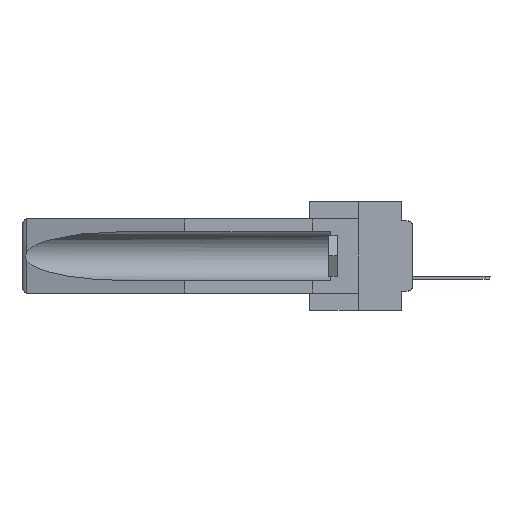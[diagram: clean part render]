
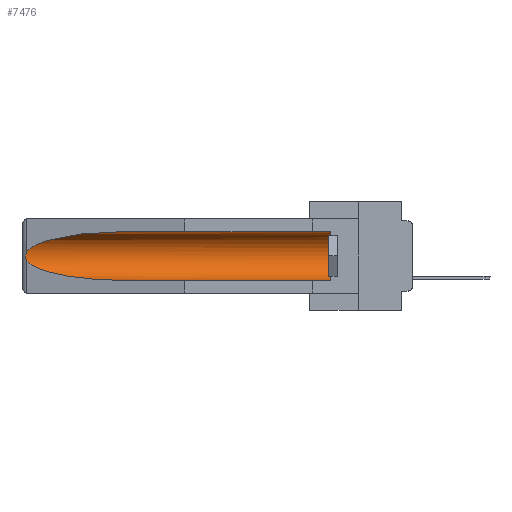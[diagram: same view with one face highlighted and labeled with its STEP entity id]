
A CAD part, left-side view. The second image highlights one B-rep face of the part: STEP entity #7476.
In plain terms, the highlighted cylindrical face has radius 2.857 mm (diameter 5.715 mm), a partial arc.
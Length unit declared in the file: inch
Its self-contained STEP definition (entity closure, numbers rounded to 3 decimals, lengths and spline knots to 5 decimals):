
#289 = VERTEX_POINT ( 'NONE', #1878 ) ;
#341 = DIRECTION ( 'NONE',  ( 0., 0., 1. ) ) ;
#725 = LINE ( 'NONE', #33284, #6023 ) ;
#1368 = ORIENTED_EDGE ( 'NONE', *, *, #16022, .T. ) ;
#1583 = EDGE_CURVE ( 'NONE', #289, #24981, #30473, .T. ) ;
#1784 = CARTESIAN_POINT ( 'NONE',  ( 0.155, 1.07973, -0.284 ) ) ;
#1878 = CARTESIAN_POINT ( 'NONE',  ( 0.155, 1.07973, -0.059 ) ) ;
#2144 = CARTESIAN_POINT ( 'NONE',  ( 0.2675, 1.53308, -0.16763 ) ) ;
#2725 = EDGE_LOOP ( 'NONE', ( #32180, #23673, #1368, #21050, #5216, #3379 ) ) ;
#2933 = EDGE_CURVE ( 'NONE', #29592, #12455, #725, .T. ) ;
#3379 = ORIENTED_EDGE ( 'NONE', *, *, #3585, .T. ) ;
#3585 = EDGE_CURVE ( 'NONE', #12005, #289, #24762, .T. ) ;
#5216 = ORIENTED_EDGE ( 'NONE', *, *, #14655, .T. ) ;
#6023 = VECTOR ( 'NONE', #20231, 39.37008 ) ;
#7077 = CARTESIAN_POINT ( 'NONE',  ( 0.155, 0.126, -0.059 ) ) ;
#7353 = CARTESIAN_POINT ( 'NONE',  ( 0.26655, 1.53094, -0.18657 ) ) ;
#7474 = CARTESIAN_POINT ( 'NONE',  ( 0.2673, 1.53269, -0.17917 ) ) ;
#7476 = ADVANCED_FACE ( 'NONE', ( #9332 ), #32379, .F. ) ;
#8204 = CARTESIAN_POINT ( 'NONE',  ( 0.155, -0.30754, -0.059 ) ) ;
#9332 = FACE_OUTER_BOUND ( 'NONE', #2725, .T. ) ;
#9966 = CARTESIAN_POINT ( 'NONE',  ( 0.26537, 1.52718, -0.14972 ) ) ;
#10027 = CARTESIAN_POINT ( 'NONE',  ( 0.26537, 1.52718, -0.14972 ) ) ;
#10951 = DIRECTION ( 'NONE',  ( 0., 1., 0. ) ) ;
#11073 = CARTESIAN_POINT ( 'NONE',  ( 0.21114, 1.30732, -0.059 ) ) ;
#11259 = CARTESIAN_POINT ( 'NONE',  ( 0.155, 1.07973, -0.284 ) ) ;
#12005 = VERTEX_POINT ( 'NONE', #7077 ) ;
#12455 = VERTEX_POINT ( 'NONE', #1784 ) ;
#12849 = AXIS2_PLACEMENT_3D ( 'NONE', #22186, #17029, #16928 ) ;
#13623 = CIRCLE ( 'NONE', #12849, 0.1125 ) ;
#13941 = CARTESIAN_POINT ( 'NONE',  ( 0.26537, 1.52718, -0.14972 ) ) ;
#14138 = CARTESIAN_POINT ( 'NONE',  ( 0.25451, 1.48313, -0.24835 ) ) ;
#14655 = EDGE_CURVE ( 'NONE', #29592, #12005, #13623, .T. ) ;
#14914 = VECTOR ( 'NONE', #10951, 39.37008 ) ;
#15169 = CARTESIAN_POINT ( 'NONE',  ( 0.26537, 1.52718, -0.19328 ) ) ;
#16022 = EDGE_CURVE ( 'NONE', #21710, #12455, #29589, .T. ) ;
#16928 = DIRECTION ( 'NONE',  ( 0., 0., 1. ) ) ;
#17029 = DIRECTION ( 'NONE',  ( 0., -1., 0. ) ) ;
#19294 = CARTESIAN_POINT ( 'NONE',  ( 0.21114, 1.30732, -0.284 ) ) ;
#19414 = CARTESIAN_POINT ( 'NONE',  ( 0.26537, 1.52718, -0.19328 ) ) ;
#20231 = DIRECTION ( 'NONE',  ( 0., 1., 0. ) ) ;
#21050 = ORIENTED_EDGE ( 'NONE', *, *, #2933, .F. ) ;
#21710 = VERTEX_POINT ( 'NONE', #25976 ) ;
#22186 = CARTESIAN_POINT ( 'NONE',  ( 0.155, 0.126, -0.1715 ) ) ;
#22338 = CARTESIAN_POINT ( 'NONE',  ( 0.155, 0.126, -0.284 ) ) ;
#22827 = B_SPLINE_CURVE_WITH_KNOTS ( 'NONE', 3,
 ( #10027, #25744, #23201, #28521, #2144, #28415, #7474, #7353, #33934, #15169 ),
 .UNSPECIFIED., .F., .F.,
 ( 4, 2, 2, 2, 4 ),
 ( 0., 0.00029, 0.00058, 0.00087, 0.00117 ),
 .UNSPECIFIED. ) ;
#23201 = CARTESIAN_POINT ( 'NONE',  ( 0.26654, 1.53092, -0.15636 ) ) ;
#23425 = AXIS2_PLACEMENT_3D ( 'NONE', #26590, #29273, #341 ) ;
#23673 = ORIENTED_EDGE ( 'NONE', *, *, #28598, .T. ) ;
#24762 = LINE ( 'NONE', #8204, #14914 ) ;
#24981 = VERTEX_POINT ( 'NONE', #9966 ) ;
#25744 = CARTESIAN_POINT ( 'NONE',  ( 0.26597, 1.52961, -0.15275 ) ) ;
#25976 = CARTESIAN_POINT ( 'NONE',  ( 0.26537, 1.52718, -0.19328 ) ) ;
#26590 = CARTESIAN_POINT ( 'NONE',  ( 0.155, -0.30754, -0.1715 ) ) ;
#28415 = CARTESIAN_POINT ( 'NONE',  ( 0.2675, 1.53308, -0.17534 ) ) ;
#28521 = CARTESIAN_POINT ( 'NONE',  ( 0.2673, 1.5327, -0.16383 ) ) ;
#28598 = EDGE_CURVE ( 'NONE', #24981, #21710, #22827, .T. ) ;
#29273 = DIRECTION ( 'NONE',  ( 0., 1., 0. ) ) ;
#29589 =( BOUNDED_CURVE ( )  B_SPLINE_CURVE ( 3, ( #19414, #14138, #19294, #11259 ),
 .UNSPECIFIED., .F., .F. ) 
 B_SPLINE_CURVE_WITH_KNOTS ( ( 4, 4 ),
 ( 0.1948, 1.5708 ),
 .UNSPECIFIED. ) 
 CURVE ( )  GEOMETRIC_REPRESENTATION_ITEM ( )  RATIONAL_B_SPLINE_CURVE ( ( 1., 0.848, 0.848, 1. ) ) 
 REPRESENTATION_ITEM ( '' )  );
#29592 = VERTEX_POINT ( 'NONE', #22338 ) ;
#29703 = CARTESIAN_POINT ( 'NONE',  ( 0.25451, 1.48313, -0.09465 ) ) ;
#30473 =( BOUNDED_CURVE ( )  B_SPLINE_CURVE ( 3, ( #31918, #11073, #29703, #13941 ),
 .UNSPECIFIED., .F., .F. ) 
 B_SPLINE_CURVE_WITH_KNOTS ( ( 4, 4 ),
 ( 4.71239, 6.08839 ),
 .UNSPECIFIED. ) 
 CURVE ( )  GEOMETRIC_REPRESENTATION_ITEM ( )  RATIONAL_B_SPLINE_CURVE ( ( 1., 0.848, 0.848, 1. ) ) 
 REPRESENTATION_ITEM ( '' )  );
#31918 = CARTESIAN_POINT ( 'NONE',  ( 0.155, 1.07973, -0.059 ) ) ;
#32180 = ORIENTED_EDGE ( 'NONE', *, *, #1583, .T. ) ;
#32379 = CYLINDRICAL_SURFACE ( 'NONE', #23425, 0.1125 ) ;
#33284 = CARTESIAN_POINT ( 'NONE',  ( 0.155, -0.30754, -0.284 ) ) ;
#33934 = CARTESIAN_POINT ( 'NONE',  ( 0.26597, 1.5296, -0.19026 ) ) ;
